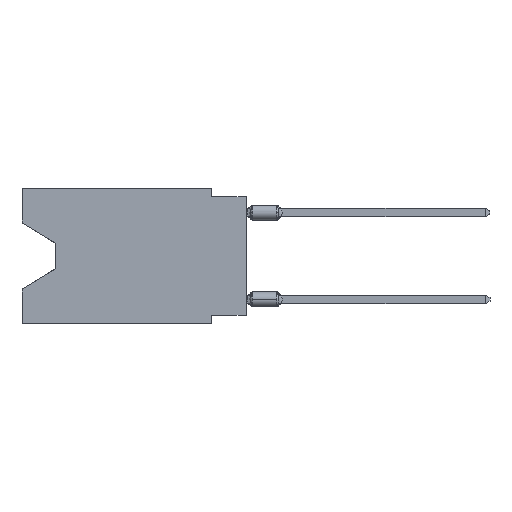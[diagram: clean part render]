
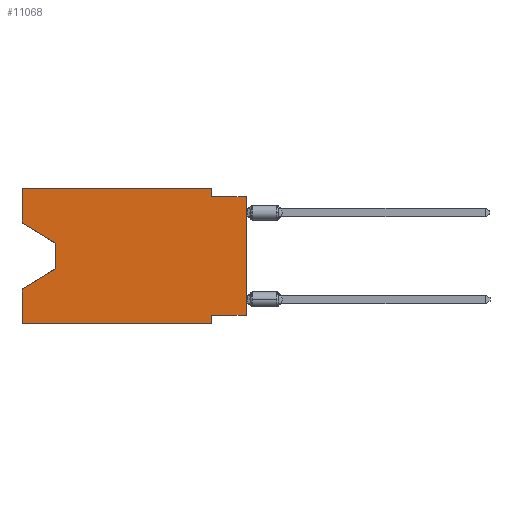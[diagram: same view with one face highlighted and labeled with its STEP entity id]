
A CAD part, left-side view. The second image highlights one B-rep face of the part: STEP entity #11068.
In plain terms, the highlighted planar face has unit normal (-1, 0, 0).
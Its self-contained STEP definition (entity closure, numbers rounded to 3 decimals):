
#522 = ORIENTED_EDGE ( 'NONE', *, *, #9797, .F. ) ;
#715 = LINE ( 'NONE', #7743, #9104 ) ;
#785 = DIRECTION ( 'NONE',  ( 0., -1., 0. ) ) ;
#801 = VERTEX_POINT ( 'NONE', #19206 ) ;
#821 = VECTOR ( 'NONE', #12763, 1000. ) ;
#989 = VERTEX_POINT ( 'NONE', #22367 ) ;
#1113 = CARTESIAN_POINT ( 'NONE',  ( 0., 2.54, -9.906 ) ) ;
#1191 = ORIENTED_EDGE ( 'NONE', *, *, #7135, .T. ) ;
#1294 = VECTOR ( 'NONE', #3610, 1000. ) ;
#1303 = EDGE_CURVE ( 'NONE', #12956, #989, #21674, .T. ) ;
#1771 = DIRECTION ( 'NONE',  ( 0., -1., 0. ) ) ;
#2128 = EDGE_CURVE ( 'NONE', #20433, #18772, #7542, .T. ) ;
#2787 = DIRECTION ( 'NONE',  ( 0., -1., 0. ) ) ;
#3009 = CARTESIAN_POINT ( 'NONE',  ( 0., 16.383, 0. ) ) ;
#3561 = EDGE_CURVE ( 'NONE', #8054, #9314, #4421, .T. ) ;
#3610 = DIRECTION ( 'NONE',  ( 0., 0., 1. ) ) ;
#3620 = LINE ( 'NONE', #19428, #19365 ) ;
#3807 = LINE ( 'NONE', #10989, #16014 ) ;
#3986 = CARTESIAN_POINT ( 'NONE',  ( 0., 16.383, -9.906 ) ) ;
#4421 = LINE ( 'NONE', #18492, #18562 ) ;
#4719 = CARTESIAN_POINT ( 'NONE',  ( 0., 2.54, 0. ) ) ;
#4847 = CARTESIAN_POINT ( 'NONE',  ( 0., 16.383, -7.36 ) ) ;
#5052 = DIRECTION ( 'NONE',  ( 0., 0., -1. ) ) ;
#5116 = EDGE_CURVE ( 'NONE', #18066, #18772, #5212, .T. ) ;
#5212 = LINE ( 'NONE', #19290, #1294 ) ;
#5253 = DIRECTION ( 'NONE',  ( 0., -0.855, -0.519 ) ) ;
#5567 = DIRECTION ( 'NONE',  ( 0., 0., -1. ) ) ;
#5619 = VECTOR ( 'NONE', #5052, 1000. ) ;
#5803 = CARTESIAN_POINT ( 'NONE',  ( 0., 16.383, 0. ) ) ;
#5897 = ORIENTED_EDGE ( 'NONE', *, *, #10301, .T. ) ;
#6991 = CARTESIAN_POINT ( 'NONE',  ( 0., 16.383, -2.546 ) ) ;
#7055 = ORIENTED_EDGE ( 'NONE', *, *, #5116, .F. ) ;
#7135 = EDGE_CURVE ( 'NONE', #8054, #7855, #20953, .T. ) ;
#7542 = LINE ( 'NONE', #21496, #821 ) ;
#7743 = CARTESIAN_POINT ( 'NONE',  ( 0., 16.383, -9.906 ) ) ;
#7855 = VERTEX_POINT ( 'NONE', #10900 ) ;
#8054 = VERTEX_POINT ( 'NONE', #15677 ) ;
#8088 = CARTESIAN_POINT ( 'NONE',  ( 0., 2.54, -9.906 ) ) ;
#8521 = ORIENTED_EDGE ( 'NONE', *, *, #22596, .F. ) ;
#8559 = LINE ( 'NONE', #15726, #8600 ) ;
#8600 = VECTOR ( 'NONE', #1771, 1000. ) ;
#8741 = EDGE_LOOP ( 'NONE', ( #1191, #5897, #19982, #7055, #19147, #18129, #21869, #14360, #8521, #22184, #522, #11878 ) ) ;
#9104 = VECTOR ( 'NONE', #2787, 1000. ) ;
#9314 = VERTEX_POINT ( 'NONE', #3009 ) ;
#9692 = VERTEX_POINT ( 'NONE', #16049 ) ;
#9733 = DIRECTION ( 'NONE',  ( 0., 0., 1. ) ) ;
#9797 = EDGE_CURVE ( 'NONE', #9314, #12956, #3807, .T. ) ;
#9944 = CARTESIAN_POINT ( 'NONE',  ( 0., 2.54, -9.271 ) ) ;
#10301 = EDGE_CURVE ( 'NONE', #7855, #20433, #14505, .T. ) ;
#10900 = CARTESIAN_POINT ( 'NONE',  ( 0., 13.97, -4.013 ) ) ;
#10985 = DIRECTION ( 'NONE',  ( 0., 0., -1. ) ) ;
#10989 = CARTESIAN_POINT ( 'NONE',  ( 0., 16.383, 0. ) ) ;
#11068 = ADVANCED_FACE ( 'NONE', ( #21367 ), #12737, .F. ) ;
#11359 = CARTESIAN_POINT ( 'NONE',  ( 0., 0., -9.271 ) ) ;
#11560 = LINE ( 'NONE', #11359, #20407 ) ;
#11878 = ORIENTED_EDGE ( 'NONE', *, *, #3561, .F. ) ;
#12353 = EDGE_CURVE ( 'NONE', #18066, #16979, #715, .T. ) ;
#12472 = VECTOR ( 'NONE', #5253, 1000. ) ;
#12713 = VECTOR ( 'NONE', #18520, 1000. ) ;
#12737 = PLANE ( 'NONE',  #13454 ) ;
#12763 = DIRECTION ( 'NONE',  ( 0., 0.855, -0.519 ) ) ;
#12853 = DIRECTION ( 'NONE',  ( 1., 0., 0. ) ) ;
#12956 = VERTEX_POINT ( 'NONE', #4719 ) ;
#12970 = VECTOR ( 'NONE', #10985, 1000. ) ;
#13454 = AXIS2_PLACEMENT_3D ( 'NONE', #5803, #12853, #5567 ) ;
#14360 = ORIENTED_EDGE ( 'NONE', *, *, #18496, .T. ) ;
#14505 = LINE ( 'NONE', #17024, #12713 ) ;
#15563 = EDGE_CURVE ( 'NONE', #801, #18865, #11560, .T. ) ;
#15677 = CARTESIAN_POINT ( 'NONE',  ( 0., 16.383, -2.546 ) ) ;
#15726 = CARTESIAN_POINT ( 'NONE',  ( 0., 0., -0.635 ) ) ;
#16014 = VECTOR ( 'NONE', #785, 1000. ) ;
#16049 = CARTESIAN_POINT ( 'NONE',  ( 0., 0., -0.635 ) ) ;
#16932 = LINE ( 'NONE', #1113, #5619 ) ;
#16979 = VERTEX_POINT ( 'NONE', #8088 ) ;
#17024 = CARTESIAN_POINT ( 'NONE',  ( 0., 13.97, -4.013 ) ) ;
#17591 = DIRECTION ( 'NONE',  ( 0., 0., 1. ) ) ;
#18066 = VERTEX_POINT ( 'NONE', #3986 ) ;
#18129 = ORIENTED_EDGE ( 'NONE', *, *, #21753, .F. ) ;
#18492 = CARTESIAN_POINT ( 'NONE',  ( 0., 16.383, 0. ) ) ;
#18496 = EDGE_CURVE ( 'NONE', #801, #9692, #3620, .T. ) ;
#18520 = DIRECTION ( 'NONE',  ( 0., 0., -1. ) ) ;
#18562 = VECTOR ( 'NONE', #9733, 1000. ) ;
#18720 = DIRECTION ( 'NONE',  ( 0., 1., 0. ) ) ;
#18772 = VERTEX_POINT ( 'NONE', #4847 ) ;
#18865 = VERTEX_POINT ( 'NONE', #9944 ) ;
#19147 = ORIENTED_EDGE ( 'NONE', *, *, #12353, .T. ) ;
#19206 = CARTESIAN_POINT ( 'NONE',  ( 0., 0., -9.271 ) ) ;
#19290 = CARTESIAN_POINT ( 'NONE',  ( 0., 16.383, 0. ) ) ;
#19365 = VECTOR ( 'NONE', #17591, 1000. ) ;
#19428 = CARTESIAN_POINT ( 'NONE',  ( 0., 0., 0. ) ) ;
#19840 = CARTESIAN_POINT ( 'NONE',  ( 0., 2.54, 0. ) ) ;
#19982 = ORIENTED_EDGE ( 'NONE', *, *, #2128, .T. ) ;
#20407 = VECTOR ( 'NONE', #18720, 1000. ) ;
#20433 = VERTEX_POINT ( 'NONE', #21780 ) ;
#20953 = LINE ( 'NONE', #6991, #12472 ) ;
#21367 = FACE_OUTER_BOUND ( 'NONE', #8741, .T. ) ;
#21496 = CARTESIAN_POINT ( 'NONE',  ( 0., 13.97, -5.893 ) ) ;
#21674 = LINE ( 'NONE', #19840, #12970 ) ;
#21753 = EDGE_CURVE ( 'NONE', #18865, #16979, #16932, .T. ) ;
#21780 = CARTESIAN_POINT ( 'NONE',  ( 0., 13.97, -5.893 ) ) ;
#21869 = ORIENTED_EDGE ( 'NONE', *, *, #15563, .F. ) ;
#22184 = ORIENTED_EDGE ( 'NONE', *, *, #1303, .F. ) ;
#22367 = CARTESIAN_POINT ( 'NONE',  ( 0., 2.54, -0.635 ) ) ;
#22596 = EDGE_CURVE ( 'NONE', #989, #9692, #8559, .T. ) ;
